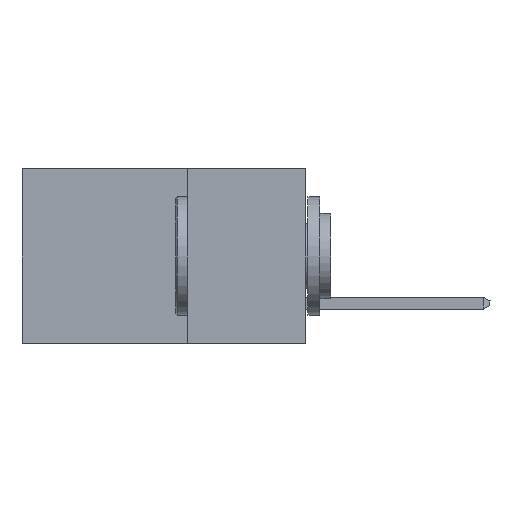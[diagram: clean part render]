
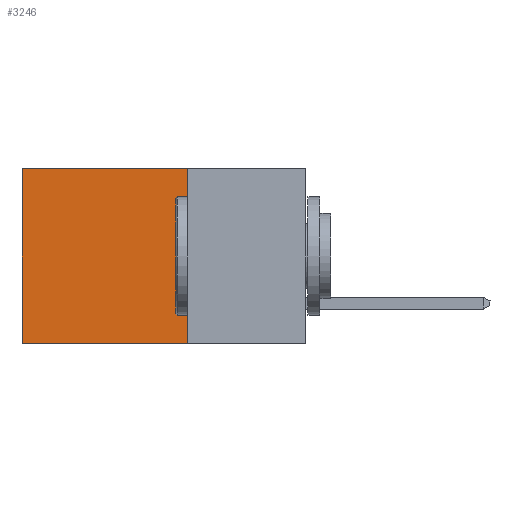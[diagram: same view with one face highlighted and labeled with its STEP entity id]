
A CAD part, left-side view. The second image highlights one B-rep face of the part: STEP entity #3246.
In plain terms, the highlighted planar face has unit normal (-1, 0, 0).
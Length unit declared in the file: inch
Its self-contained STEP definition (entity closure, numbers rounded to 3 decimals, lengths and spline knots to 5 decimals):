
#369 = VECTOR ( 'NONE', #3919, 39.37008 ) ;
#577 = AXIS2_PLACEMENT_3D ( 'NONE', #11521, #6635, #4615 ) ;
#590 = PLANE ( 'NONE',  #577 ) ;
#706 = VERTEX_POINT ( 'NONE', #922 ) ;
#922 = CARTESIAN_POINT ( 'NONE',  ( 0.2615, 0.25, 0. ) ) ;
#1269 = LINE ( 'NONE', #1977, #5840 ) ;
#1977 = CARTESIAN_POINT ( 'NONE',  ( 0.2615, 0.25, -0.37 ) ) ;
#3246 = ADVANCED_FACE ( 'NONE', ( #12698 ), #590, .F. ) ;
#3493 = ORIENTED_EDGE ( 'NONE', *, *, #12660, .F. ) ;
#3558 = EDGE_CURVE ( 'NONE', #11649, #5485, #5376, .T. ) ;
#3919 = DIRECTION ( 'NONE',  ( 0., 1., 0. ) ) ;
#4404 = DIRECTION ( 'NONE',  ( 0., 0., -1. ) ) ;
#4615 = DIRECTION ( 'NONE',  ( 0., 0., -1. ) ) ;
#5079 = ORIENTED_EDGE ( 'NONE', *, *, #3558, .T. ) ;
#5376 = LINE ( 'NONE', #7395, #7428 ) ;
#5485 = VERTEX_POINT ( 'NONE', #11427 ) ;
#5840 = VECTOR ( 'NONE', #5947, 39.37008 ) ;
#5947 = DIRECTION ( 'NONE',  ( 0., 0., -1. ) ) ;
#6229 = VERTEX_POINT ( 'NONE', #10045 ) ;
#6635 = DIRECTION ( 'NONE',  ( 1., 0., 0. ) ) ;
#6736 = ORIENTED_EDGE ( 'NONE', *, *, #9244, .F. ) ;
#6766 = CARTESIAN_POINT ( 'NONE',  ( 0.2615, 0.6, 0. ) ) ;
#6840 = CARTESIAN_POINT ( 'NONE',  ( 0.2615, 0.25, 0. ) ) ;
#6919 = LINE ( 'NONE', #12847, #369 ) ;
#7395 = CARTESIAN_POINT ( 'NONE',  ( 0.2615, 0.6, -0.37 ) ) ;
#7428 = VECTOR ( 'NONE', #4404, 39.37008 ) ;
#8456 = VECTOR ( 'NONE', #10822, 39.37008 ) ;
#9244 = EDGE_CURVE ( 'NONE', #706, #6229, #1269, .T. ) ;
#9774 = EDGE_LOOP ( 'NONE', ( #5079, #3493, #6736, #11325 ) ) ;
#9775 = LINE ( 'NONE', #6840, #8456 ) ;
#10045 = CARTESIAN_POINT ( 'NONE',  ( 0.2615, 0.25, -0.37 ) ) ;
#10822 = DIRECTION ( 'NONE',  ( 0., 1., 0. ) ) ;
#11325 = ORIENTED_EDGE ( 'NONE', *, *, #11766, .T. ) ;
#11427 = CARTESIAN_POINT ( 'NONE',  ( 0.2615, 0.6, -0.37 ) ) ;
#11521 = CARTESIAN_POINT ( 'NONE',  ( 0.2615, 0.25, -0.37 ) ) ;
#11649 = VERTEX_POINT ( 'NONE', #6766 ) ;
#11766 = EDGE_CURVE ( 'NONE', #706, #11649, #9775, .T. ) ;
#12660 = EDGE_CURVE ( 'NONE', #6229, #5485, #6919, .T. ) ;
#12698 = FACE_OUTER_BOUND ( 'NONE', #9774, .T. ) ;
#12847 = CARTESIAN_POINT ( 'NONE',  ( 0.2615, 0.25, -0.37 ) ) ;
